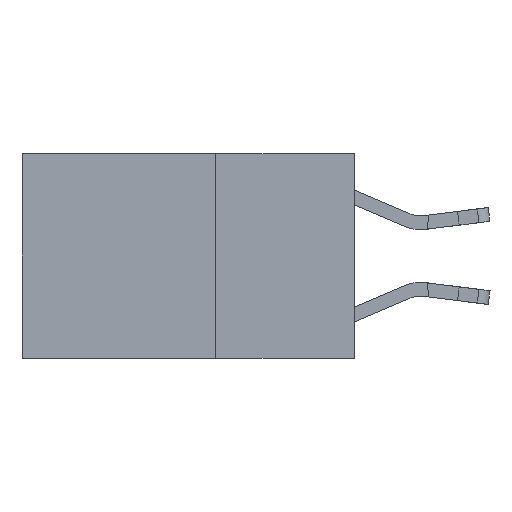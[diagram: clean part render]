
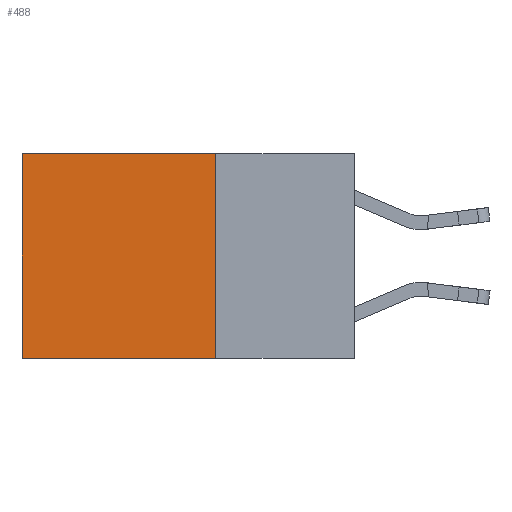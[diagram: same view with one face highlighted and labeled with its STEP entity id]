
A CAD part, left-side view. The second image highlights one B-rep face of the part: STEP entity #488.
In plain terms, the highlighted planar face has unit normal (-1, 0, 0).
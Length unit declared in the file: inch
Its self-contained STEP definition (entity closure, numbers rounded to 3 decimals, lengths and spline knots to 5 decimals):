
#488 = ADVANCED_FACE ( 'NONE', ( #2611 ), #10306, .F. ) ;
#839 = EDGE_LOOP ( 'NONE', ( #1953, #2913, #5657, #3253 ) ) ;
#893 = DIRECTION ( 'NONE',  ( 0., 0., -1. ) ) ;
#1313 = CARTESIAN_POINT ( 'NONE',  ( 0.2625, 0.25, 0. ) ) ;
#1618 = CARTESIAN_POINT ( 'NONE',  ( 0.2625, 0.25, 0. ) ) ;
#1702 = VERTEX_POINT ( 'NONE', #9300 ) ;
#1908 = DIRECTION ( 'NONE',  ( 0., 0., -1. ) ) ;
#1953 = ORIENTED_EDGE ( 'NONE', *, *, #12397, .T. ) ;
#2404 = EDGE_CURVE ( 'NONE', #6707, #7311, #10173, .T. ) ;
#2429 = VECTOR ( 'NONE', #893, 39.37008 ) ;
#2581 = LINE ( 'NONE', #11303, #9704 ) ;
#2611 = FACE_OUTER_BOUND ( 'NONE', #839, .T. ) ;
#2913 = ORIENTED_EDGE ( 'NONE', *, *, #6198, .F. ) ;
#3253 = ORIENTED_EDGE ( 'NONE', *, *, #9334, .T. ) ;
#4296 = CARTESIAN_POINT ( 'NONE',  ( 0.2625, 0.25, 0. ) ) ;
#4356 = CARTESIAN_POINT ( 'NONE',  ( 0.2625, 0.25, -0.37 ) ) ;
#5032 = CARTESIAN_POINT ( 'NONE',  ( 0.2625, 0.6, 0. ) ) ;
#5319 = DIRECTION ( 'NONE',  ( 1., 0., 0. ) ) ;
#5657 = ORIENTED_EDGE ( 'NONE', *, *, #2404, .F. ) ;
#5984 = CARTESIAN_POINT ( 'NONE',  ( 0.2625, 0.25, 0. ) ) ;
#6006 = VECTOR ( 'NONE', #12676, 39.37008 ) ;
#6198 = EDGE_CURVE ( 'NONE', #7311, #1702, #2581, .T. ) ;
#6331 = LINE ( 'NONE', #1618, #6006 ) ;
#6365 = LINE ( 'NONE', #10004, #8702 ) ;
#6500 = VERTEX_POINT ( 'NONE', #5032 ) ;
#6707 = VERTEX_POINT ( 'NONE', #1313 ) ;
#7311 = VERTEX_POINT ( 'NONE', #4356 ) ;
#8219 = DIRECTION ( 'NONE',  ( 0., 1., 0. ) ) ;
#8702 = VECTOR ( 'NONE', #1908, 39.37008 ) ;
#9300 = CARTESIAN_POINT ( 'NONE',  ( 0.2625, 0.6, -0.37 ) ) ;
#9334 = EDGE_CURVE ( 'NONE', #6707, #6500, #6331, .T. ) ;
#9704 = VECTOR ( 'NONE', #8219, 39.37008 ) ;
#9742 = AXIS2_PLACEMENT_3D ( 'NONE', #4296, #5319, #12312 ) ;
#10004 = CARTESIAN_POINT ( 'NONE',  ( 0.2625, 0.6, 0. ) ) ;
#10173 = LINE ( 'NONE', #5984, #2429 ) ;
#10306 = PLANE ( 'NONE',  #9742 ) ;
#11303 = CARTESIAN_POINT ( 'NONE',  ( 0.2625, 0.25, -0.37 ) ) ;
#12312 = DIRECTION ( 'NONE',  ( 0., 0., -1. ) ) ;
#12397 = EDGE_CURVE ( 'NONE', #6500, #1702, #6365, .T. ) ;
#12676 = DIRECTION ( 'NONE',  ( 0., 1., 0. ) ) ;
